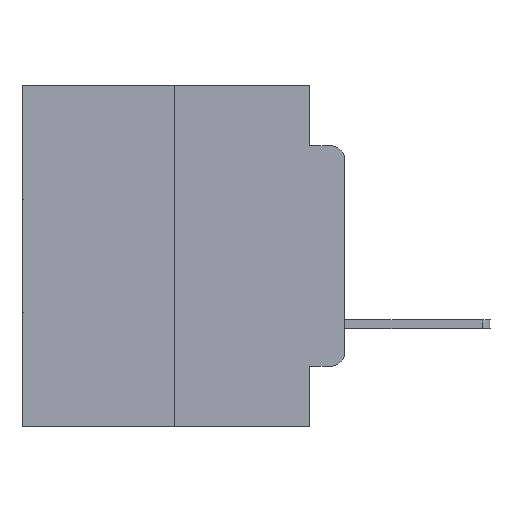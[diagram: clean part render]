
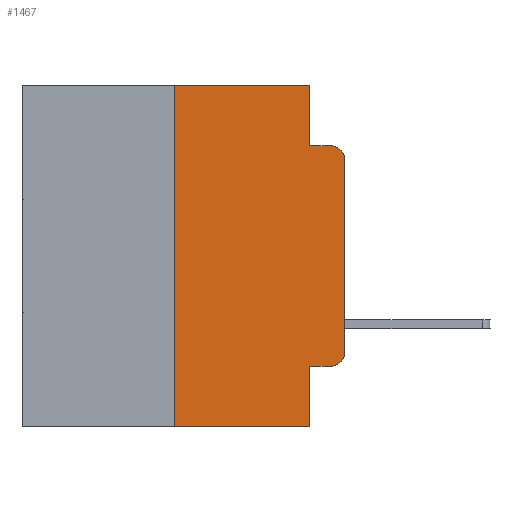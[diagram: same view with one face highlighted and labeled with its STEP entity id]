
A CAD part, left-side view. The second image highlights one B-rep face of the part: STEP entity #1467.
In plain terms, the highlighted planar face has unit normal (-1, 0, 0).
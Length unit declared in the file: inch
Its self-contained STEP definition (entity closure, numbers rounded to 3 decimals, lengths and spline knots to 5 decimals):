
#962 = CARTESIAN_POINT ( 'NONE',  ( 0., 0.25, 0. ) ) ;
#1451 = DIRECTION ( 'NONE',  ( -1., 0., 0. ) ) ;
#1467 = ADVANCED_FACE ( 'NONE', ( #2564 ), #20146, .F. ) ;
#1735 = AXIS2_PLACEMENT_3D ( 'NONE', #13953, #1451, #16020 ) ;
#2564 = FACE_OUTER_BOUND ( 'NONE', #25432, .T. ) ;
#3036 = DIRECTION ( 'NONE',  ( 0., 0., 1. ) ) ;
#3222 = AXIS2_PLACEMENT_3D ( 'NONE', #20035, #19970, #19953 ) ;
#3495 = DIRECTION ( 'NONE',  ( 0., -1., 0. ) ) ;
#3499 = DIRECTION ( 'NONE',  ( 0., -1., 0. ) ) ;
#3650 = VERTEX_POINT ( 'NONE', #18279 ) ;
#3768 = VECTOR ( 'NONE', #11165, 39.37008 ) ;
#5180 = LINE ( 'NONE', #22000, #10745 ) ;
#5267 = CARTESIAN_POINT ( 'NONE',  ( 0., 0.051, 0. ) ) ;
#5665 = CARTESIAN_POINT ( 'NONE',  ( 0., 0.02, -0.0885 ) ) ;
#5739 = VECTOR ( 'NONE', #15317, 39.37008 ) ;
#6792 = ORIENTED_EDGE ( 'NONE', *, *, #25875, .T. ) ;
#7090 = CARTESIAN_POINT ( 'NONE',  ( 0., 0.473, -0.5 ) ) ;
#7506 = VERTEX_POINT ( 'NONE', #5267 ) ;
#8113 = EDGE_CURVE ( 'NONE', #20041, #23389, #5180, .T. ) ;
#8403 = VECTOR ( 'NONE', #10471, 39.37008 ) ;
#8755 = ORIENTED_EDGE ( 'NONE', *, *, #9941, .T. ) ;
#9056 = DIRECTION ( 'NONE',  ( 0., 0., -1. ) ) ;
#9152 = CARTESIAN_POINT ( 'NONE',  ( 0., 0.051, -0.4115 ) ) ;
#9185 = CARTESIAN_POINT ( 'NONE',  ( 0., 0., 0. ) ) ;
#9308 = VERTEX_POINT ( 'NONE', #9152 ) ;
#9497 = EDGE_CURVE ( 'NONE', #10173, #7506, #15543, .T. ) ;
#9750 = ORIENTED_EDGE ( 'NONE', *, *, #11409, .T. ) ;
#9941 = EDGE_CURVE ( 'NONE', #25160, #12774, #20254, .T. ) ;
#10173 = VERTEX_POINT ( 'NONE', #22225 ) ;
#10249 = CARTESIAN_POINT ( 'NONE',  ( 0., 0.02, -0.4115 ) ) ;
#10266 = VERTEX_POINT ( 'NONE', #10249 ) ;
#10471 = DIRECTION ( 'NONE',  ( 0., -1., 0. ) ) ;
#10745 = VECTOR ( 'NONE', #3499, 39.37008 ) ;
#10793 = DIRECTION ( 'NONE',  ( 0., 0., -1. ) ) ;
#11165 = DIRECTION ( 'NONE',  ( 0., -1., 0. ) ) ;
#11198 = DIRECTION ( 'NONE',  ( -1., 0., 0. ) ) ;
#11223 = CIRCLE ( 'NONE', #18517, 0.02 ) ;
#11409 = EDGE_CURVE ( 'NONE', #21373, #23389, #22116, .T. ) ;
#11864 = LINE ( 'NONE', #21297, #22712 ) ;
#12335 = ORIENTED_EDGE ( 'NONE', *, *, #15217, .T. ) ;
#12468 = ORIENTED_EDGE ( 'NONE', *, *, #8113, .F. ) ;
#12774 = VERTEX_POINT ( 'NONE', #22590 ) ;
#13953 = CARTESIAN_POINT ( 'NONE',  ( 0., 0.02, -0.1085 ) ) ;
#14553 = EDGE_CURVE ( 'NONE', #9308, #12774, #17128, .T. ) ;
#14651 = CARTESIAN_POINT ( 'NONE',  ( 0., 0.051, -0.4115 ) ) ;
#14909 = ORIENTED_EDGE ( 'NONE', *, *, #15913, .F. ) ;
#15217 = EDGE_CURVE ( 'NONE', #3650, #21373, #17412, .T. ) ;
#15317 = DIRECTION ( 'NONE',  ( 0., 0., 1. ) ) ;
#15543 = LINE ( 'NONE', #25919, #25622 ) ;
#15773 = VECTOR ( 'NONE', #3036, 39.37008 ) ;
#15913 = EDGE_CURVE ( 'NONE', #25160, #10173, #21796, .T. ) ;
#16020 = DIRECTION ( 'NONE',  ( 0., 0., -1. ) ) ;
#17128 = LINE ( 'NONE', #20994, #21873 ) ;
#17412 = LINE ( 'NONE', #9185, #5739 ) ;
#18279 = CARTESIAN_POINT ( 'NONE',  ( 0., 0., -0.3915 ) ) ;
#18517 = AXIS2_PLACEMENT_3D ( 'NONE', #23403, #11198, #25424 ) ;
#18715 = CARTESIAN_POINT ( 'NONE',  ( 0., 0.25, -0.5 ) ) ;
#19034 = ORIENTED_EDGE ( 'NONE', *, *, #14553, .F. ) ;
#19323 = LINE ( 'NONE', #14651, #8403 ) ;
#19953 = DIRECTION ( 'NONE',  ( 0., 0., -1. ) ) ;
#19970 = DIRECTION ( 'NONE',  ( 1., 0., 0. ) ) ;
#20035 = CARTESIAN_POINT ( 'NONE',  ( 0., 0.473, 0. ) ) ;
#20041 = VERTEX_POINT ( 'NONE', #21349 ) ;
#20146 = PLANE ( 'NONE',  #3222 ) ;
#20204 = CARTESIAN_POINT ( 'NONE',  ( 0., 0., -0.1085 ) ) ;
#20254 = LINE ( 'NONE', #7090, #3768 ) ;
#20994 = CARTESIAN_POINT ( 'NONE',  ( 0., 0.051, 0. ) ) ;
#21297 = CARTESIAN_POINT ( 'NONE',  ( 0., 0.051, 0. ) ) ;
#21349 = CARTESIAN_POINT ( 'NONE',  ( 0., 0.051, -0.0885 ) ) ;
#21373 = VERTEX_POINT ( 'NONE', #20204 ) ;
#21796 = LINE ( 'NONE', #962, #15773 ) ;
#21873 = VECTOR ( 'NONE', #10793, 39.37008 ) ;
#22000 = CARTESIAN_POINT ( 'NONE',  ( 0., 0.051, -0.0885 ) ) ;
#22055 = ORIENTED_EDGE ( 'NONE', *, *, #25859, .F. ) ;
#22116 = CIRCLE ( 'NONE', #1735, 0.02 ) ;
#22225 = CARTESIAN_POINT ( 'NONE',  ( 0., 0.25, 0. ) ) ;
#22590 = CARTESIAN_POINT ( 'NONE',  ( 0., 0.051, -0.5 ) ) ;
#22712 = VECTOR ( 'NONE', #9056, 39.37008 ) ;
#23126 = ORIENTED_EDGE ( 'NONE', *, *, #24555, .T. ) ;
#23389 = VERTEX_POINT ( 'NONE', #5665 ) ;
#23403 = CARTESIAN_POINT ( 'NONE',  ( 0., 0.02, -0.3915 ) ) ;
#24555 = EDGE_CURVE ( 'NONE', #9308, #10266, #19323, .T. ) ;
#25160 = VERTEX_POINT ( 'NONE', #18715 ) ;
#25424 = DIRECTION ( 'NONE',  ( 0., 0., -1. ) ) ;
#25432 = EDGE_LOOP ( 'NONE', ( #12335, #9750, #12468, #22055, #26244, #14909, #8755, #19034, #23126, #6792 ) ) ;
#25622 = VECTOR ( 'NONE', #3495, 39.37008 ) ;
#25859 = EDGE_CURVE ( 'NONE', #7506, #20041, #11864, .T. ) ;
#25875 = EDGE_CURVE ( 'NONE', #10266, #3650, #11223, .T. ) ;
#25919 = CARTESIAN_POINT ( 'NONE',  ( 0., 0.473, 0. ) ) ;
#26244 = ORIENTED_EDGE ( 'NONE', *, *, #9497, .F. ) ;
